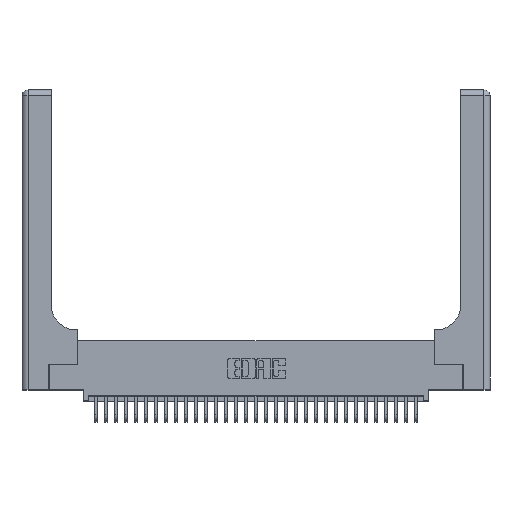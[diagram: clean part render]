
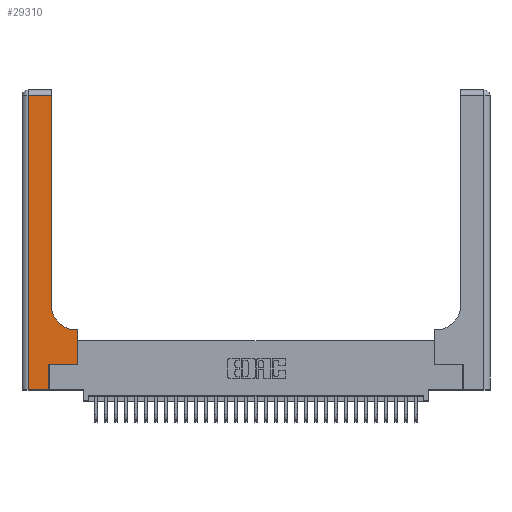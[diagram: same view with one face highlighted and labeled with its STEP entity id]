
A CAD part, top view. The second image highlights one B-rep face of the part: STEP entity #29310.
In plain terms, the highlighted planar face has unit normal (0, 0, 1).
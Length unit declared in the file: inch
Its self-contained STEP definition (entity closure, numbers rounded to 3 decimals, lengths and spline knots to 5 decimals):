
#997 = CARTESIAN_POINT ( 'NONE',  ( 0.269, 0., 0.37 ) ) ;
#1198 = EDGE_CURVE ( 'NONE', #12772, #32134, #29897, .T. ) ;
#1339 = ORIENTED_EDGE ( 'NONE', *, *, #25330, .T. ) ;
#1462 = VECTOR ( 'NONE', #19224, 39.37008 ) ;
#1740 = VERTEX_POINT ( 'NONE', #13447 ) ;
#2001 = EDGE_CURVE ( 'NONE', #6480, #12772, #3078, .T. ) ;
#2113 = ORIENTED_EDGE ( 'NONE', *, *, #20105, .T. ) ;
#3078 = LINE ( 'NONE', #20353, #11316 ) ;
#3130 = EDGE_LOOP ( 'NONE', ( #17689, #1339, #21410, #20029, #6741, #28215, #31300, #2113, #11403 ) ) ;
#3567 = CARTESIAN_POINT ( 'NONE',  ( 0.5415, 0.85, 0.37 ) ) ;
#4441 = EDGE_CURVE ( 'NONE', #1740, #11261, #14913, .T. ) ;
#4615 = DIRECTION ( 'NONE',  ( -1., 0., 0. ) ) ;
#5251 = CIRCLE ( 'NONE', #26805, 0.25 ) ;
#6480 = VERTEX_POINT ( 'NONE', #31356 ) ;
#6741 = ORIENTED_EDGE ( 'NONE', *, *, #1198, .T. ) ;
#7569 = CARTESIAN_POINT ( 'NONE',  ( 0.5585, 0.25, 0.37 ) ) ;
#8036 = VERTEX_POINT ( 'NONE', #14370 ) ;
#8440 = CARTESIAN_POINT ( 'NONE',  ( 0.2915, 2.94, 0.37 ) ) ;
#9814 = PLANE ( 'NONE',  #31089 ) ;
#10150 = VECTOR ( 'NONE', #29567, 39.37008 ) ;
#10195 = EDGE_CURVE ( 'NONE', #20136, #6480, #26893, .T. ) ;
#10321 = DIRECTION ( 'NONE',  ( 1., 0., 0. ) ) ;
#10577 = DIRECTION ( 'NONE',  ( 0., 1., 0. ) ) ;
#11261 = VERTEX_POINT ( 'NONE', #8440 ) ;
#11316 = VECTOR ( 'NONE', #10321, 39.37008 ) ;
#11403 = ORIENTED_EDGE ( 'NONE', *, *, #16984, .T. ) ;
#11506 = DIRECTION ( 'NONE',  ( 0., 0., -1. ) ) ;
#12455 = LINE ( 'NONE', #17698, #27273 ) ;
#12673 = DIRECTION ( 'NONE',  ( 0., 0., -1. ) ) ;
#12772 = VERTEX_POINT ( 'NONE', #997 ) ;
#13079 = CARTESIAN_POINT ( 'NONE',  ( 0.269, 0.25, 0.37 ) ) ;
#13447 = CARTESIAN_POINT ( 'NONE',  ( 0.2915, 0.85, 0.37 ) ) ;
#13493 = CARTESIAN_POINT ( 'NONE',  ( 0.269, 0., 0.37 ) ) ;
#14156 = LINE ( 'NONE', #20961, #21557 ) ;
#14370 = CARTESIAN_POINT ( 'NONE',  ( 0.5415, 0.6, 0.37 ) ) ;
#14835 = VECTOR ( 'NONE', #17141, 39.37008 ) ;
#14913 = LINE ( 'NONE', #17404, #30914 ) ;
#15054 = CARTESIAN_POINT ( 'NONE',  ( 0.5585, 0.6, 0.37 ) ) ;
#15241 = CARTESIAN_POINT ( 'NONE',  ( 0., 3., 0.37 ) ) ;
#16984 = EDGE_CURVE ( 'NONE', #8036, #1740, #5251, .T. ) ;
#17141 = DIRECTION ( 'NONE',  ( -1., 0., 0. ) ) ;
#17404 = CARTESIAN_POINT ( 'NONE',  ( 0.2915, 3., 0.37 ) ) ;
#17689 = ORIENTED_EDGE ( 'NONE', *, *, #4441, .T. ) ;
#17698 = CARTESIAN_POINT ( 'NONE',  ( 0.2915, 0.6, 0.37 ) ) ;
#19224 = DIRECTION ( 'NONE',  ( 1., 0., 0. ) ) ;
#19544 = CARTESIAN_POINT ( 'NONE',  ( 0., 2.94, 0.37 ) ) ;
#19924 = VECTOR ( 'NONE', #23179, 39.37008 ) ;
#20029 = ORIENTED_EDGE ( 'NONE', *, *, #2001, .T. ) ;
#20105 = EDGE_CURVE ( 'NONE', #22220, #8036, #12455, .T. ) ;
#20136 = VERTEX_POINT ( 'NONE', #25418 ) ;
#20353 = CARTESIAN_POINT ( 'NONE',  ( 0., 0., 0.37 ) ) ;
#20961 = CARTESIAN_POINT ( 'NONE',  ( 0.5585, 0.25, 0.37 ) ) ;
#21410 = ORIENTED_EDGE ( 'NONE', *, *, #10195, .T. ) ;
#21557 = VECTOR ( 'NONE', #10577, 39.37008 ) ;
#22220 = VERTEX_POINT ( 'NONE', #15054 ) ;
#22375 = VERTEX_POINT ( 'NONE', #7569 ) ;
#23179 = DIRECTION ( 'NONE',  ( 0., -1., 0. ) ) ;
#24412 = CARTESIAN_POINT ( 'NONE',  ( 0.269, 0.25, 0.37 ) ) ;
#25330 = EDGE_CURVE ( 'NONE', #11261, #20136, #26744, .T. ) ;
#25418 = CARTESIAN_POINT ( 'NONE',  ( 0.06, 2.94, 0.37 ) ) ;
#26424 = EDGE_CURVE ( 'NONE', #32134, #22375, #27394, .T. ) ;
#26744 = LINE ( 'NONE', #19544, #14835 ) ;
#26805 = AXIS2_PLACEMENT_3D ( 'NONE', #3567, #11506, #32788 ) ;
#26893 = LINE ( 'NONE', #28546, #19924 ) ;
#27273 = VECTOR ( 'NONE', #33443, 39.37008 ) ;
#27394 = LINE ( 'NONE', #24412, #1462 ) ;
#28215 = ORIENTED_EDGE ( 'NONE', *, *, #26424, .T. ) ;
#28546 = CARTESIAN_POINT ( 'NONE',  ( 0.06, 3., 0.37 ) ) ;
#29310 = ADVANCED_FACE ( 'NONE', ( #33388 ), #9814, .F. ) ;
#29567 = DIRECTION ( 'NONE',  ( 0., 1., 0. ) ) ;
#29897 = LINE ( 'NONE', #13493, #10150 ) ;
#30914 = VECTOR ( 'NONE', #32894, 39.37008 ) ;
#31089 = AXIS2_PLACEMENT_3D ( 'NONE', #15241, #12673, #4615 ) ;
#31300 = ORIENTED_EDGE ( 'NONE', *, *, #32931, .T. ) ;
#31356 = CARTESIAN_POINT ( 'NONE',  ( 0.06, 0., 0.37 ) ) ;
#32134 = VERTEX_POINT ( 'NONE', #13079 ) ;
#32788 = DIRECTION ( 'NONE',  ( 1., 0., 0. ) ) ;
#32894 = DIRECTION ( 'NONE',  ( 0., 1., 0. ) ) ;
#32931 = EDGE_CURVE ( 'NONE', #22375, #22220, #14156, .T. ) ;
#33388 = FACE_OUTER_BOUND ( 'NONE', #3130, .T. ) ;
#33443 = DIRECTION ( 'NONE',  ( -1., 0., 0. ) ) ;
